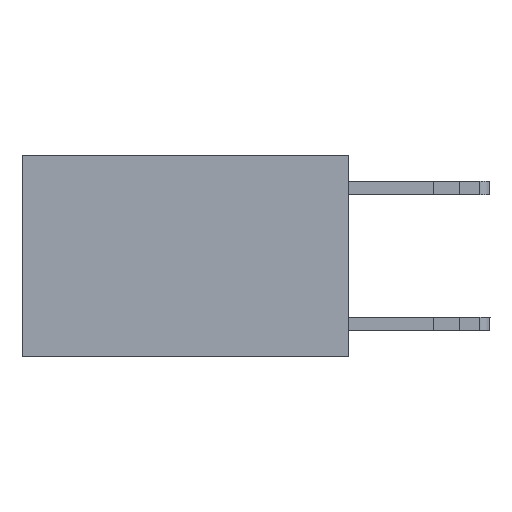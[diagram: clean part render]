
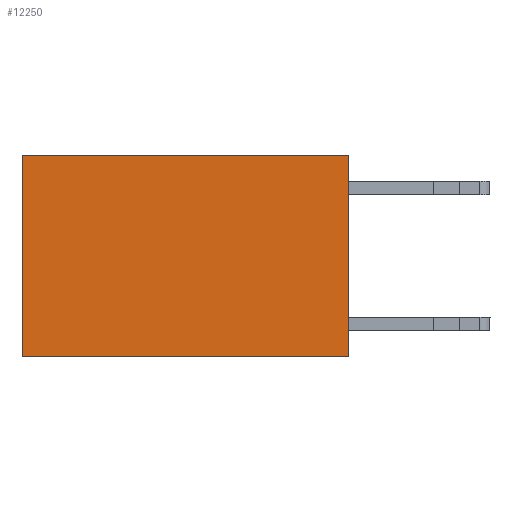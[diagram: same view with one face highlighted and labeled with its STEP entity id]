
A CAD part, left-side view. The second image highlights one B-rep face of the part: STEP entity #12250.
In plain terms, the highlighted planar face has unit normal (-1, 0, 0).
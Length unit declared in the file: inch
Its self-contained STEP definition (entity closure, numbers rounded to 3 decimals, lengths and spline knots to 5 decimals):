
#801 = PLANE ( 'NONE',  #16816 ) ;
#1321 = VERTEX_POINT ( 'NONE', #17808 ) ;
#1388 = EDGE_LOOP ( 'NONE', ( #3485, #7480, #7687, #3397 ) ) ;
#2309 = EDGE_CURVE ( 'NONE', #7284, #1321, #19681, .T. ) ;
#2425 = EDGE_CURVE ( 'NONE', #7284, #8572, #13775, .T. ) ;
#2845 = EDGE_CURVE ( 'NONE', #1321, #6347, #10660, .T. ) ;
#3397 = ORIENTED_EDGE ( 'NONE', *, *, #2309, .T. ) ;
#3443 = VECTOR ( 'NONE', #18797, 39.37008 ) ;
#3485 = ORIENTED_EDGE ( 'NONE', *, *, #2845, .T. ) ;
#4661 = EDGE_CURVE ( 'NONE', #8572, #6347, #14176, .T. ) ;
#4681 = CARTESIAN_POINT ( 'NONE',  ( 0.2625, 0.6, 0. ) ) ;
#4767 = CARTESIAN_POINT ( 'NONE',  ( 0.2625, 0., -0.37 ) ) ;
#5486 = DIRECTION ( 'NONE',  ( 0., 0., -1. ) ) ;
#6347 = VERTEX_POINT ( 'NONE', #11586 ) ;
#7284 = VERTEX_POINT ( 'NONE', #18178 ) ;
#7480 = ORIENTED_EDGE ( 'NONE', *, *, #4661, .F. ) ;
#7687 = ORIENTED_EDGE ( 'NONE', *, *, #2425, .F. ) ;
#8572 = VERTEX_POINT ( 'NONE', #4767 ) ;
#9703 = CARTESIAN_POINT ( 'NONE',  ( 0.2625, 0., 0. ) ) ;
#10660 = LINE ( 'NONE', #4681, #17796 ) ;
#10823 = DIRECTION ( 'NONE',  ( 0., 0., -1. ) ) ;
#11586 = CARTESIAN_POINT ( 'NONE',  ( 0.2625, 0.6, -0.37 ) ) ;
#11614 = CARTESIAN_POINT ( 'NONE',  ( 0.2625, 0., 0. ) ) ;
#12250 = ADVANCED_FACE ( 'NONE', ( #17217 ), #801, .F. ) ;
#12955 = DIRECTION ( 'NONE',  ( 0., 0., -1. ) ) ;
#13225 = DIRECTION ( 'NONE',  ( 0., 1., 0. ) ) ;
#13309 = VECTOR ( 'NONE', #12955, 39.37008 ) ;
#13775 = LINE ( 'NONE', #14498, #13309 ) ;
#14176 = LINE ( 'NONE', #19241, #17720 ) ;
#14498 = CARTESIAN_POINT ( 'NONE',  ( 0.2625, 0., 0. ) ) ;
#14668 = DIRECTION ( 'NONE',  ( 1., 0., 0. ) ) ;
#16816 = AXIS2_PLACEMENT_3D ( 'NONE', #11614, #14668, #5486 ) ;
#17217 = FACE_OUTER_BOUND ( 'NONE', #1388, .T. ) ;
#17720 = VECTOR ( 'NONE', #13225, 39.37008 ) ;
#17796 = VECTOR ( 'NONE', #10823, 39.37008 ) ;
#17808 = CARTESIAN_POINT ( 'NONE',  ( 0.2625, 0.6, 0. ) ) ;
#18178 = CARTESIAN_POINT ( 'NONE',  ( 0.2625, 0., 0. ) ) ;
#18797 = DIRECTION ( 'NONE',  ( 0., 1., 0. ) ) ;
#19241 = CARTESIAN_POINT ( 'NONE',  ( 0.2625, 0., -0.37 ) ) ;
#19681 = LINE ( 'NONE', #9703, #3443 ) ;
